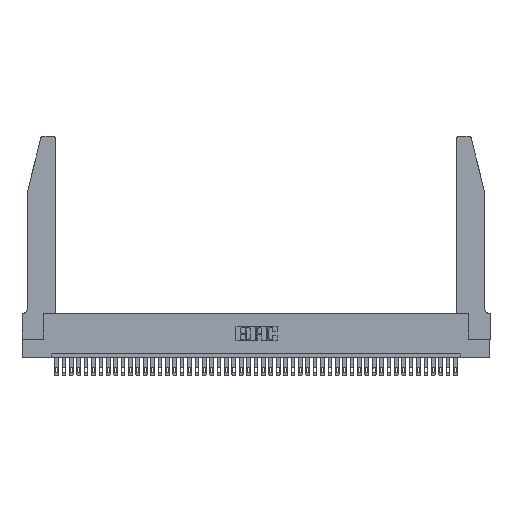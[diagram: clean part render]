
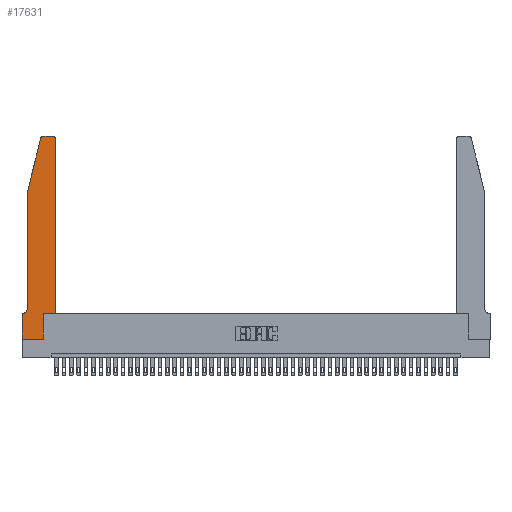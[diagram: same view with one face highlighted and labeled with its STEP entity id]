
A CAD part, top view. The second image highlights one B-rep face of the part: STEP entity #17631.
In plain terms, the highlighted planar face has unit normal (0, 0, 1).
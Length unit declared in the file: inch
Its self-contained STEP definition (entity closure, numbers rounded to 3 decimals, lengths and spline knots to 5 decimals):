
#745 = CARTESIAN_POINT ( 'NONE',  ( 0.0755, 2., 0.37 ) ) ;
#771 = DIRECTION ( 'NONE',  ( 0., -1., 0. ) ) ;
#1893 = VECTOR ( 'NONE', #39083, 39.37008 ) ;
#2369 = ORIENTED_EDGE ( 'NONE', *, *, #20668, .T. ) ;
#3046 = CIRCLE ( 'NONE', #43778, 0.03 ) ;
#3799 = PLANE ( 'NONE',  #38166 ) ;
#4180 = VERTEX_POINT ( 'NONE', #12202 ) ;
#4653 = VERTEX_POINT ( 'NONE', #13576 ) ;
#5260 = DIRECTION ( 'NONE',  ( 0., 0., 1. ) ) ;
#6071 = ORIENTED_EDGE ( 'NONE', *, *, #37996, .T. ) ;
#6495 = DIRECTION ( 'NONE',  ( 1., 0., 0. ) ) ;
#6917 = VECTOR ( 'NONE', #7786, 39.37008 ) ;
#7320 = EDGE_CURVE ( 'NONE', #22719, #30941, #13391, .T. ) ;
#7786 = DIRECTION ( 'NONE',  ( -0.239, -0.971, 0. ) ) ;
#7996 = DIRECTION ( 'NONE',  ( -1., 0., 0. ) ) ;
#8254 = LINE ( 'NONE', #38224, #35091 ) ;
#8589 = AXIS2_PLACEMENT_3D ( 'NONE', #29939, #18999, #26048 ) ;
#8907 = ORIENTED_EDGE ( 'NONE', *, *, #28131, .T. ) ;
#9226 = VECTOR ( 'NONE', #6495, 39.37008 ) ;
#11979 = DIRECTION ( 'NONE',  ( 1., 0., 0. ) ) ;
#12202 = CARTESIAN_POINT ( 'NONE',  ( 0., 0.35, 0.37 ) ) ;
#13391 = LINE ( 'NONE', #745, #6917 ) ;
#13576 = CARTESIAN_POINT ( 'NONE',  ( 0.284, 2.75, 0.37 ) ) ;
#14296 = CARTESIAN_POINT ( 'NONE',  ( 0.4205, 2.75, 0.37 ) ) ;
#14655 = EDGE_CURVE ( 'NONE', #26952, #20479, #36039, .T. ) ;
#14691 = VECTOR ( 'NONE', #29937, 39.37008 ) ;
#15115 = DIRECTION ( 'NONE',  ( 0., 0., 1. ) ) ;
#16498 = CARTESIAN_POINT ( 'NONE',  ( 0.0755, 2., 0.37 ) ) ;
#16619 = EDGE_CURVE ( 'NONE', #41560, #20690, #24092, .T. ) ;
#16892 = ORIENTED_EDGE ( 'NONE', *, *, #34361, .T. ) ;
#17197 = DIRECTION ( 'NONE',  ( 0., 1., 0. ) ) ;
#17631 = ADVANCED_FACE ( 'NONE', ( #37373 ), #3799, .T. ) ;
#17961 = LINE ( 'NONE', #35811, #1893 ) ;
#18999 = DIRECTION ( 'NONE',  ( 0., 0., 1. ) ) ;
#19890 = DIRECTION ( 'NONE',  ( -1., 0., 0. ) ) ;
#20479 = VERTEX_POINT ( 'NONE', #26558 ) ;
#20668 = EDGE_CURVE ( 'NONE', #39937, #4653, #42351, .T. ) ;
#20690 = VERTEX_POINT ( 'NONE', #29039 ) ;
#20729 = EDGE_LOOP ( 'NONE', ( #2369, #8907, #32882, #44062, #40737, #24028, #16892, #6071, #27769, #35849, #20745, #41093 ) ) ;
#20745 = ORIENTED_EDGE ( 'NONE', *, *, #36191, .T. ) ;
#20913 = CARTESIAN_POINT ( 'NONE',  ( 0.4505, 0.35, 0.37 ) ) ;
#22254 = EDGE_CURVE ( 'NONE', #31579, #39937, #35801, .T. ) ;
#22719 = VERTEX_POINT ( 'NONE', #28943 ) ;
#22750 = LINE ( 'NONE', #39943, #14691 ) ;
#22951 = CARTESIAN_POINT ( 'NONE',  ( 0.2865, 0.35, 0.37 ) ) ;
#24028 = ORIENTED_EDGE ( 'NONE', *, *, #28863, .T. ) ;
#24092 = CIRCLE ( 'NONE', #24427, 0.07 ) ;
#24427 = AXIS2_PLACEMENT_3D ( 'NONE', #31384, #38702, #7996 ) ;
#24463 = CARTESIAN_POINT ( 'NONE',  ( 0., 0.35, 0.37 ) ) ;
#24607 = CARTESIAN_POINT ( 'NONE',  ( 0.2605, 2.75, 0.37 ) ) ;
#24715 = VECTOR ( 'NONE', #19890, 39.37008 ) ;
#25800 = CARTESIAN_POINT ( 'NONE',  ( 0.284, 2.72, 0.37 ) ) ;
#26048 = DIRECTION ( 'NONE',  ( 1., 0., 0. ) ) ;
#26421 = LINE ( 'NONE', #20913, #40883 ) ;
#26558 = CARTESIAN_POINT ( 'NONE',  ( 0.4505, 0.35, 0.37 ) ) ;
#26952 = VERTEX_POINT ( 'NONE', #22951 ) ;
#27210 = VERTEX_POINT ( 'NONE', #30439 ) ;
#27267 = CARTESIAN_POINT ( 'NONE',  ( 0.0755, 0.42, 0.37 ) ) ;
#27321 = CARTESIAN_POINT ( 'NONE',  ( 0.4505, 0.35, 0.37 ) ) ;
#27761 = CARTESIAN_POINT ( 'NONE',  ( 0., 0., 0.37 ) ) ;
#27769 = ORIENTED_EDGE ( 'NONE', *, *, #28085, .T. ) ;
#28085 = EDGE_CURVE ( 'NONE', #27210, #26952, #17961, .T. ) ;
#28131 = EDGE_CURVE ( 'NONE', #4653, #22719, #3046, .T. ) ;
#28157 = EDGE_CURVE ( 'NONE', #30941, #41560, #33590, .T. ) ;
#28320 = VECTOR ( 'NONE', #44164, 39.37008 ) ;
#28863 = EDGE_CURVE ( 'NONE', #20690, #4180, #22750, .T. ) ;
#28943 = CARTESIAN_POINT ( 'NONE',  ( 0.25487, 2.72718, 0.37 ) ) ;
#29039 = CARTESIAN_POINT ( 'NONE',  ( 0.0055, 0.35, 0.37 ) ) ;
#29429 = LINE ( 'NONE', #40710, #28320 ) ;
#29937 = DIRECTION ( 'NONE',  ( -1., 0., 0. ) ) ;
#29939 = CARTESIAN_POINT ( 'NONE',  ( 0.4205, 2.72, 0.37 ) ) ;
#30439 = CARTESIAN_POINT ( 'NONE',  ( 0.2865, 0., 0.37 ) ) ;
#30941 = VERTEX_POINT ( 'NONE', #16498 ) ;
#31384 = CARTESIAN_POINT ( 'NONE',  ( 0.0055, 0.42, 0.37 ) ) ;
#31579 = VERTEX_POINT ( 'NONE', #34664 ) ;
#31630 = VERTEX_POINT ( 'NONE', #27761 ) ;
#32882 = ORIENTED_EDGE ( 'NONE', *, *, #7320, .T. ) ;
#33590 = LINE ( 'NONE', #39701, #43152 ) ;
#34361 = EDGE_CURVE ( 'NONE', #4180, #31630, #8254, .T. ) ;
#34664 = CARTESIAN_POINT ( 'NONE',  ( 0.4505, 2.72, 0.37 ) ) ;
#35091 = VECTOR ( 'NONE', #771, 39.37008 ) ;
#35801 = CIRCLE ( 'NONE', #8589, 0.03 ) ;
#35811 = CARTESIAN_POINT ( 'NONE',  ( 0.2865, 0.35, 0.37 ) ) ;
#35849 = ORIENTED_EDGE ( 'NONE', *, *, #14655, .T. ) ;
#36039 = LINE ( 'NONE', #27321, #9226 ) ;
#36191 = EDGE_CURVE ( 'NONE', #20479, #31579, #26421, .T. ) ;
#37373 = FACE_OUTER_BOUND ( 'NONE', #20729, .T. ) ;
#37996 = EDGE_CURVE ( 'NONE', #31630, #27210, #29429, .T. ) ;
#38166 = AXIS2_PLACEMENT_3D ( 'NONE', #24463, #15115, #39071 ) ;
#38224 = CARTESIAN_POINT ( 'NONE',  ( 0., 0., 0.37 ) ) ;
#38702 = DIRECTION ( 'NONE',  ( 0., 0., -1. ) ) ;
#39071 = DIRECTION ( 'NONE',  ( 1., 0., 0. ) ) ;
#39083 = DIRECTION ( 'NONE',  ( 0., 1., 0. ) ) ;
#39701 = CARTESIAN_POINT ( 'NONE',  ( 0.0755, 2., 0.37 ) ) ;
#39937 = VERTEX_POINT ( 'NONE', #14296 ) ;
#39943 = CARTESIAN_POINT ( 'NONE',  ( 0.0755, 0.35, 0.37 ) ) ;
#40710 = CARTESIAN_POINT ( 'NONE',  ( 0., 0., 0.37 ) ) ;
#40737 = ORIENTED_EDGE ( 'NONE', *, *, #16619, .T. ) ;
#40883 = VECTOR ( 'NONE', #17197, 39.37008 ) ;
#41093 = ORIENTED_EDGE ( 'NONE', *, *, #22254, .T. ) ;
#41560 = VERTEX_POINT ( 'NONE', #27267 ) ;
#42351 = LINE ( 'NONE', #24607, #24715 ) ;
#43002 = DIRECTION ( 'NONE',  ( 0., -1., 0. ) ) ;
#43152 = VECTOR ( 'NONE', #43002, 39.37008 ) ;
#43778 = AXIS2_PLACEMENT_3D ( 'NONE', #25800, #5260, #11979 ) ;
#44062 = ORIENTED_EDGE ( 'NONE', *, *, #28157, .T. ) ;
#44164 = DIRECTION ( 'NONE',  ( 1., 0., 0. ) ) ;
